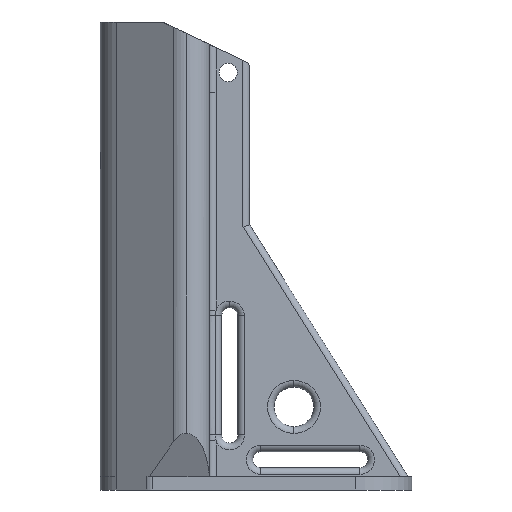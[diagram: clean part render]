
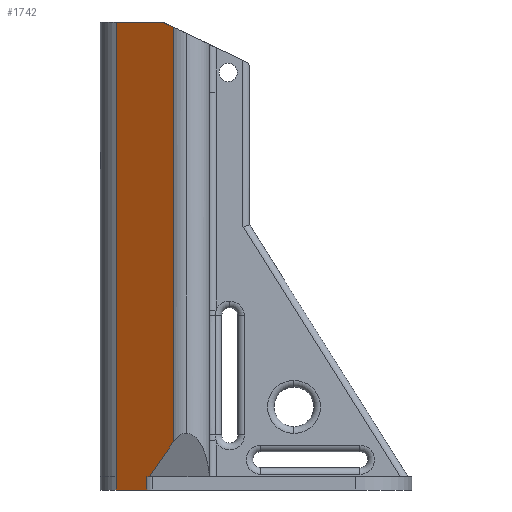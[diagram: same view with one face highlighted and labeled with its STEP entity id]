
A CAD part, left-side view. The second image highlights one B-rep face of the part: STEP entity #1742.
In plain terms, the highlighted planar face has unit normal (-0.828, 0.561, 0).
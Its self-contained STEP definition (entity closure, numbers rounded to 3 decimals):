
#20 = DIRECTION ( 'NONE',  ( 0.828, -0.561, 0. ) ) ;
#111 = LINE ( 'NONE', #4749, #2923 ) ;
#137 = VECTOR ( 'NONE', #1506, 1000. ) ;
#177 = ORIENTED_EDGE ( 'NONE', *, *, #3257, .F. ) ;
#241 = CARTESIAN_POINT ( 'NONE',  ( -13.121, 35.779, 174.625 ) ) ;
#421 = DIRECTION ( 'NONE',  ( 0.561, 0.828, 0. ) ) ;
#433 = DIRECTION ( 'NONE',  ( -0.522, -0.77, -0.367 ) ) ;
#438 = CARTESIAN_POINT ( 'NONE',  ( -27.968, 13.878, 174.625 ) ) ;
#501 = CARTESIAN_POINT ( 'NONE',  ( -25.107, 18.098, 174.625 ) ) ;
#524 = EDGE_CURVE ( 'NONE', #810, #2209, #4207, .T. ) ;
#586 = VERTEX_POINT ( 'NONE', #501 ) ;
#637 = ORIENTED_EDGE ( 'NONE', *, *, #3291, .F. ) ;
#644 = ORIENTED_EDGE ( 'NONE', *, *, #3951, .F. ) ;
#652 = VERTEX_POINT ( 'NONE', #3942 ) ;
#654 = VECTOR ( 'NONE', #3117, 1000. ) ;
#766 = VERTEX_POINT ( 'NONE', #3865 ) ;
#810 = VERTEX_POINT ( 'NONE', #2827 ) ;
#813 = DIRECTION ( 'NONE',  ( 0.359, 0.529, -0.769 ) ) ;
#873 = LINE ( 'NONE', #3107, #1113 ) ;
#875 = LINE ( 'NONE', #3387, #2785 ) ;
#970 = VERTEX_POINT ( 'NONE', #2215 ) ;
#1042 = LINE ( 'NONE', #3776, #137 ) ;
#1083 = DIRECTION ( 'NONE',  ( 0.561, 0.828, 0. ) ) ;
#1113 = VECTOR ( 'NONE', #813, 1000. ) ;
#1155 = EDGE_CURVE ( 'NONE', #3806, #586, #1042, .T. ) ;
#1214 = ORIENTED_EDGE ( 'NONE', *, *, #1155, .F. ) ;
#1216 = CARTESIAN_POINT ( 'NONE',  ( -25.107, 18.098, 174.625 ) ) ;
#1224 = EDGE_CURVE ( 'NONE', #2008, #3405, #1561, .T. ) ;
#1311 = ORIENTED_EDGE ( 'NONE', *, *, #4830, .F. ) ;
#1506 = DIRECTION ( 'NONE',  ( -0.561, -0.828, 0. ) ) ;
#1561 = LINE ( 'NONE', #438, #654 ) ;
#1665 = ORIENTED_EDGE ( 'NONE', *, *, #524, .F. ) ;
#1704 = ORIENTED_EDGE ( 'NONE', *, *, #1814, .F. ) ;
#1714 = CARTESIAN_POINT ( 'NONE',  ( -13.121, 35.779, 174.625 ) ) ;
#1742 = ADVANCED_FACE ( 'NONE', ( #2573 ), #2300, .F. ) ;
#1781 = VECTOR ( 'NONE', #4370, 1000. ) ;
#1814 = EDGE_CURVE ( 'NONE', #586, #2008, #3638, .T. ) ;
#1920 = CARTESIAN_POINT ( 'NONE',  ( -25.608, 17.36, 174.625 ) ) ;
#2008 = VERTEX_POINT ( 'NONE', #2938 ) ;
#2209 = VERTEX_POINT ( 'NONE', #4598 ) ;
#2215 = CARTESIAN_POINT ( 'NONE',  ( -13.121, 35.779, 0. ) ) ;
#2300 = PLANE ( 'NONE',  #4891 ) ;
#2362 = ORIENTED_EDGE ( 'NONE', *, *, #1224, .F. ) ;
#2379 = EDGE_LOOP ( 'NONE', ( #1214, #3206, #637, #644, #177, #1665, #1311, #2362, #1704 ) ) ;
#2573 = FACE_OUTER_BOUND ( 'NONE', #2379, .T. ) ;
#2687 = DIRECTION ( 'NONE',  ( 0.561, 0.828, 0. ) ) ;
#2706 = CARTESIAN_POINT ( 'NONE',  ( -25.608, 17.36, 0. ) ) ;
#2785 = VECTOR ( 'NONE', #1083, 1000. ) ;
#2799 = LINE ( 'NONE', #241, #4582 ) ;
#2827 = CARTESIAN_POINT ( 'NONE',  ( -21.717, 23.099, 0. ) ) ;
#2921 = DIRECTION ( 'NONE',  ( 0., 0., 1. ) ) ;
#2923 = VECTOR ( 'NONE', #3597, 1000. ) ;
#2938 = CARTESIAN_POINT ( 'NONE',  ( -27.968, 13.878, 172.616 ) ) ;
#3107 = CARTESIAN_POINT ( 'NONE',  ( -27.968, 13.878, 13.405 ) ) ;
#3117 = DIRECTION ( 'NONE',  ( 0., 0., -1. ) ) ;
#3206 = ORIENTED_EDGE ( 'NONE', *, *, #3343, .F. ) ;
#3210 = VECTOR ( 'NONE', #421, 1000. ) ;
#3257 = EDGE_CURVE ( 'NONE', #2209, #652, #111, .T. ) ;
#3291 = EDGE_CURVE ( 'NONE', #766, #970, #4834, .T. ) ;
#3343 = EDGE_CURVE ( 'NONE', #970, #3806, #2799, .T. ) ;
#3387 = CARTESIAN_POINT ( 'NONE',  ( -25.608, 17.36, -5.08 ) ) ;
#3405 = VERTEX_POINT ( 'NONE', #3735 ) ;
#3597 = DIRECTION ( 'NONE',  ( 0., 0., -1. ) ) ;
#3638 = LINE ( 'NONE', #1216, #4403 ) ;
#3735 = CARTESIAN_POINT ( 'NONE',  ( -27.968, 13.878, 13.405 ) ) ;
#3776 = CARTESIAN_POINT ( 'NONE',  ( -13.121, 35.779, 174.625 ) ) ;
#3806 = VERTEX_POINT ( 'NONE', #4451 ) ;
#3865 = CARTESIAN_POINT ( 'NONE',  ( -13.121, 35.779, -5.08 ) ) ;
#3942 = CARTESIAN_POINT ( 'NONE',  ( -21.061, 24.067, -5.08 ) ) ;
#3951 = EDGE_CURVE ( 'NONE', #652, #766, #875, .T. ) ;
#4207 = LINE ( 'NONE', #2706, #3210 ) ;
#4370 = DIRECTION ( 'NONE',  ( 0., 0., 1. ) ) ;
#4403 = VECTOR ( 'NONE', #433, 1000. ) ;
#4451 = CARTESIAN_POINT ( 'NONE',  ( -13.121, 35.779, 174.625 ) ) ;
#4582 = VECTOR ( 'NONE', #2921, 1000. ) ;
#4598 = CARTESIAN_POINT ( 'NONE',  ( -21.061, 24.067, 0. ) ) ;
#4749 = CARTESIAN_POINT ( 'NONE',  ( -21.061, 24.067, 174.625 ) ) ;
#4830 = EDGE_CURVE ( 'NONE', #3405, #810, #873, .T. ) ;
#4834 = LINE ( 'NONE', #1714, #1781 ) ;
#4891 = AXIS2_PLACEMENT_3D ( 'NONE', #1920, #20, #2687 ) ;
